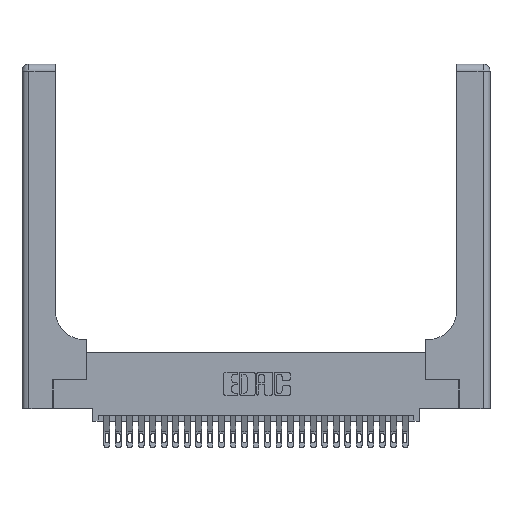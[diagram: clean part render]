
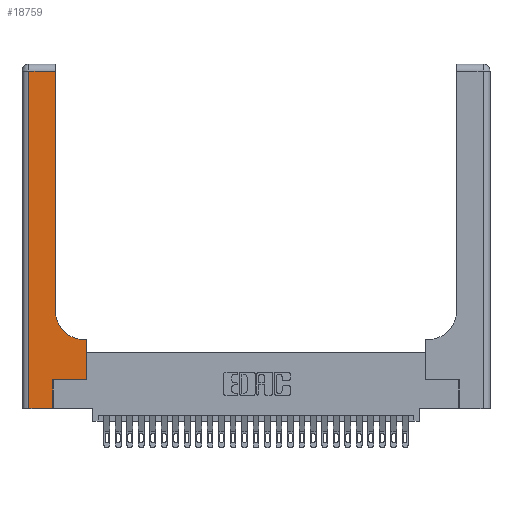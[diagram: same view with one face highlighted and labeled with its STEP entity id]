
A CAD part, top view. The second image highlights one B-rep face of the part: STEP entity #18759.
In plain terms, the highlighted planar face has unit normal (0, 0, 1).
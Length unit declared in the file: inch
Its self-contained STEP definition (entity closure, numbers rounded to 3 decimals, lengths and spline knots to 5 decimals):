
#81 = EDGE_CURVE ( 'NONE', #20089, #3543, #8782, .T. ) ;
#451 = VERTEX_POINT ( 'NONE', #11607 ) ;
#952 = LINE ( 'NONE', #18156, #17317 ) ;
#1058 = EDGE_CURVE ( 'NONE', #4741, #20089, #9756, .T. ) ;
#1462 = VERTEX_POINT ( 'NONE', #9768 ) ;
#1608 = VERTEX_POINT ( 'NONE', #15040 ) ;
#2133 = CARTESIAN_POINT ( 'NONE',  ( 0.2915, 0.85, 0.37 ) ) ;
#2771 = VERTEX_POINT ( 'NONE', #28761 ) ;
#2981 = EDGE_CURVE ( 'NONE', #2771, #12661, #15589, .T. ) ;
#3059 = ORIENTED_EDGE ( 'NONE', *, *, #1058, .T. ) ;
#3105 = EDGE_CURVE ( 'NONE', #12661, #1462, #952, .T. ) ;
#3543 = VERTEX_POINT ( 'NONE', #2133 ) ;
#4536 = VECTOR ( 'NONE', #24500, 39.37008 ) ;
#4741 = VERTEX_POINT ( 'NONE', #14290 ) ;
#4949 = CARTESIAN_POINT ( 'NONE',  ( 0.269, 0.25, 0.37 ) ) ;
#5254 = ORIENTED_EDGE ( 'NONE', *, *, #2981, .T. ) ;
#5265 = CARTESIAN_POINT ( 'NONE',  ( 0., 3., 0.37 ) ) ;
#5362 = DIRECTION ( 'NONE',  ( 0., 0., -1. ) ) ;
#5461 = PLANE ( 'NONE',  #12320 ) ;
#6686 = ORIENTED_EDGE ( 'NONE', *, *, #19597, .T. ) ;
#7161 = LINE ( 'NONE', #7472, #9609 ) ;
#7392 = EDGE_CURVE ( 'NONE', #1608, #24256, #7711, .T. ) ;
#7472 = CARTESIAN_POINT ( 'NONE',  ( 0., 0., 0.37 ) ) ;
#7711 = LINE ( 'NONE', #20707, #23025 ) ;
#8059 = DIRECTION ( 'NONE',  ( 0., -1., 0. ) ) ;
#8413 = CARTESIAN_POINT ( 'NONE',  ( 0.5415, 0.6, 0.37 ) ) ;
#8741 = ORIENTED_EDGE ( 'NONE', *, *, #7392, .T. ) ;
#8782 = CIRCLE ( 'NONE', #10169, 0.25 ) ;
#8912 = CARTESIAN_POINT ( 'NONE',  ( 0.2915, 0.6, 0.37 ) ) ;
#9609 = VECTOR ( 'NONE', #11666, 39.37008 ) ;
#9718 = DIRECTION ( 'NONE',  ( 1., 0., 0. ) ) ;
#9756 = LINE ( 'NONE', #8912, #27534 ) ;
#9768 = CARTESIAN_POINT ( 'NONE',  ( 0.06, 0., 0.37 ) ) ;
#10169 = AXIS2_PLACEMENT_3D ( 'NONE', #12572, #17046, #28353 ) ;
#10828 = EDGE_CURVE ( 'NONE', #451, #4741, #13329, .T. ) ;
#11475 = EDGE_LOOP ( 'NONE', ( #6686, #5254, #26971, #15228, #8741, #27604, #20383, #3059, #12345 ) ) ;
#11607 = CARTESIAN_POINT ( 'NONE',  ( 0.5585, 0.25, 0.37 ) ) ;
#11666 = DIRECTION ( 'NONE',  ( 1., 0., 0. ) ) ;
#12034 = CARTESIAN_POINT ( 'NONE',  ( 0.06, 2.94, 0.37 ) ) ;
#12151 = DIRECTION ( 'NONE',  ( 0., 1., 0. ) ) ;
#12320 = AXIS2_PLACEMENT_3D ( 'NONE', #5265, #5362, #25417 ) ;
#12345 = ORIENTED_EDGE ( 'NONE', *, *, #81, .T. ) ;
#12572 = CARTESIAN_POINT ( 'NONE',  ( 0.5415, 0.85, 0.37 ) ) ;
#12661 = VERTEX_POINT ( 'NONE', #12034 ) ;
#13329 = LINE ( 'NONE', #26887, #23784 ) ;
#14118 = CARTESIAN_POINT ( 'NONE',  ( 0.269, 0.25, 0.37 ) ) ;
#14290 = CARTESIAN_POINT ( 'NONE',  ( 0.5585, 0.6, 0.37 ) ) ;
#15040 = CARTESIAN_POINT ( 'NONE',  ( 0.269, 0., 0.37 ) ) ;
#15206 = DIRECTION ( 'NONE',  ( -1., 0., 0. ) ) ;
#15228 = ORIENTED_EDGE ( 'NONE', *, *, #16117, .T. ) ;
#15589 = LINE ( 'NONE', #26572, #20125 ) ;
#16117 = EDGE_CURVE ( 'NONE', #1462, #1608, #7161, .T. ) ;
#16530 = VECTOR ( 'NONE', #9718, 39.37008 ) ;
#17046 = DIRECTION ( 'NONE',  ( 0., 0., -1. ) ) ;
#17317 = VECTOR ( 'NONE', #8059, 39.37008 ) ;
#18156 = CARTESIAN_POINT ( 'NONE',  ( 0.06, 3., 0.37 ) ) ;
#18759 = ADVANCED_FACE ( 'NONE', ( #20958 ), #5461, .F. ) ;
#19597 = EDGE_CURVE ( 'NONE', #3543, #2771, #21291, .T. ) ;
#20089 = VERTEX_POINT ( 'NONE', #8413 ) ;
#20125 = VECTOR ( 'NONE', #15206, 39.37008 ) ;
#20383 = ORIENTED_EDGE ( 'NONE', *, *, #10828, .T. ) ;
#20707 = CARTESIAN_POINT ( 'NONE',  ( 0.269, 0., 0.37 ) ) ;
#20958 = FACE_OUTER_BOUND ( 'NONE', #11475, .T. ) ;
#21291 = LINE ( 'NONE', #24587, #4536 ) ;
#23025 = VECTOR ( 'NONE', #12151, 39.37008 ) ;
#23784 = VECTOR ( 'NONE', #24829, 39.37008 ) ;
#24256 = VERTEX_POINT ( 'NONE', #14118 ) ;
#24500 = DIRECTION ( 'NONE',  ( 0., 1., 0. ) ) ;
#24587 = CARTESIAN_POINT ( 'NONE',  ( 0.2915, 3., 0.37 ) ) ;
#24829 = DIRECTION ( 'NONE',  ( 0., 1., 0. ) ) ;
#25028 = EDGE_CURVE ( 'NONE', #24256, #451, #25569, .T. ) ;
#25417 = DIRECTION ( 'NONE',  ( -1., 0., 0. ) ) ;
#25569 = LINE ( 'NONE', #4949, #16530 ) ;
#26572 = CARTESIAN_POINT ( 'NONE',  ( 0., 2.94, 0.37 ) ) ;
#26887 = CARTESIAN_POINT ( 'NONE',  ( 0.5585, 0.25, 0.37 ) ) ;
#26971 = ORIENTED_EDGE ( 'NONE', *, *, #3105, .T. ) ;
#27413 = DIRECTION ( 'NONE',  ( -1., 0., 0. ) ) ;
#27534 = VECTOR ( 'NONE', #27413, 39.37008 ) ;
#27604 = ORIENTED_EDGE ( 'NONE', *, *, #25028, .T. ) ;
#28353 = DIRECTION ( 'NONE',  ( 1., 0., 0. ) ) ;
#28761 = CARTESIAN_POINT ( 'NONE',  ( 0.2915, 2.94, 0.37 ) ) ;
